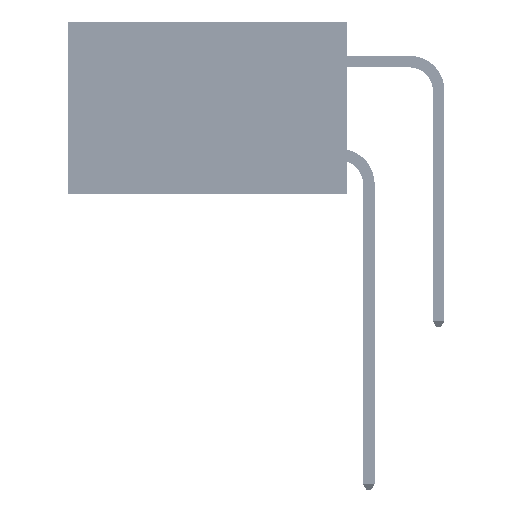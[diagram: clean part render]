
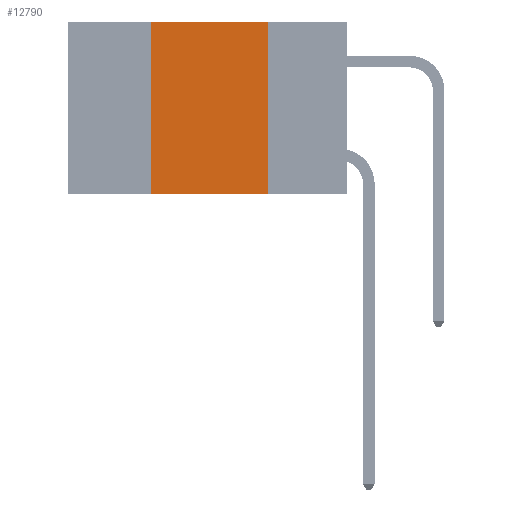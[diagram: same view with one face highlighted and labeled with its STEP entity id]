
A CAD part, left-side view. The second image highlights one B-rep face of the part: STEP entity #12790.
In plain terms, the highlighted planar face has unit normal (-1, 0, 0).
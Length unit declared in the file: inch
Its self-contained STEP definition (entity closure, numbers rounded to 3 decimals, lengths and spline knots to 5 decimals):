
#194 = CARTESIAN_POINT ( 'NONE',  ( 0., 0.6, 0. ) ) ;
#196 = VECTOR ( 'NONE', #20275, 39.37008 ) ;
#374 = DIRECTION ( 'NONE',  ( 0., 0., -1. ) ) ;
#618 = VERTEX_POINT ( 'NONE', #29048 ) ;
#6970 = EDGE_CURVE ( 'NONE', #28247, #16361, #21543, .T. ) ;
#9179 = VERTEX_POINT ( 'NONE', #39043 ) ;
#11541 = CARTESIAN_POINT ( 'NONE',  ( 0., 0.6, 0. ) ) ;
#12790 = ADVANCED_FACE ( 'NONE', ( #45274 ), #13083, .F. ) ;
#13083 = PLANE ( 'NONE',  #19802 ) ;
#14090 = LINE ( 'NONE', #24239, #33920 ) ;
#15735 = LINE ( 'NONE', #11541, #35541 ) ;
#16361 = VERTEX_POINT ( 'NONE', #37684 ) ;
#17191 = EDGE_CURVE ( 'NONE', #618, #9179, #15735, .T. ) ;
#19540 = ORIENTED_EDGE ( 'NONE', *, *, #35120, .F. ) ;
#19802 = AXIS2_PLACEMENT_3D ( 'NONE', #194, #25835, #374 ) ;
#20012 = DIRECTION ( 'NONE',  ( 0., 0., 1. ) ) ;
#20275 = DIRECTION ( 'NONE',  ( 0., -1., 0. ) ) ;
#21543 = LINE ( 'NONE', #41305, #196 ) ;
#24239 = CARTESIAN_POINT ( 'NONE',  ( 0., 0.42, 0. ) ) ;
#24815 = LINE ( 'NONE', #27842, #34713 ) ;
#25835 = DIRECTION ( 'NONE',  ( 1., 0., 0. ) ) ;
#27842 = CARTESIAN_POINT ( 'NONE',  ( 0., 0.17, 0. ) ) ;
#28247 = VERTEX_POINT ( 'NONE', #51759 ) ;
#29048 = CARTESIAN_POINT ( 'NONE',  ( 0., 0.42, 0. ) ) ;
#33920 = VECTOR ( 'NONE', #20012, 39.37008 ) ;
#34099 = ORIENTED_EDGE ( 'NONE', *, *, #50558, .F. ) ;
#34713 = VECTOR ( 'NONE', #53104, 39.37008 ) ;
#35120 = EDGE_CURVE ( 'NONE', #28247, #618, #14090, .T. ) ;
#35541 = VECTOR ( 'NONE', #45371, 39.37008 ) ;
#37684 = CARTESIAN_POINT ( 'NONE',  ( 0., 0.17, -0.37 ) ) ;
#39043 = CARTESIAN_POINT ( 'NONE',  ( 0., 0.17, 0. ) ) ;
#41305 = CARTESIAN_POINT ( 'NONE',  ( 0., 0.6, -0.37 ) ) ;
#45274 = FACE_OUTER_BOUND ( 'NONE', #54624, .T. ) ;
#45371 = DIRECTION ( 'NONE',  ( 0., -1., 0. ) ) ;
#45982 = ORIENTED_EDGE ( 'NONE', *, *, #6970, .T. ) ;
#49308 = ORIENTED_EDGE ( 'NONE', *, *, #17191, .F. ) ;
#50558 = EDGE_CURVE ( 'NONE', #9179, #16361, #24815, .T. ) ;
#51759 = CARTESIAN_POINT ( 'NONE',  ( 0., 0.42, -0.37 ) ) ;
#53104 = DIRECTION ( 'NONE',  ( 0., 0., -1. ) ) ;
#54624 = EDGE_LOOP ( 'NONE', ( #34099, #49308, #19540, #45982 ) ) ;
